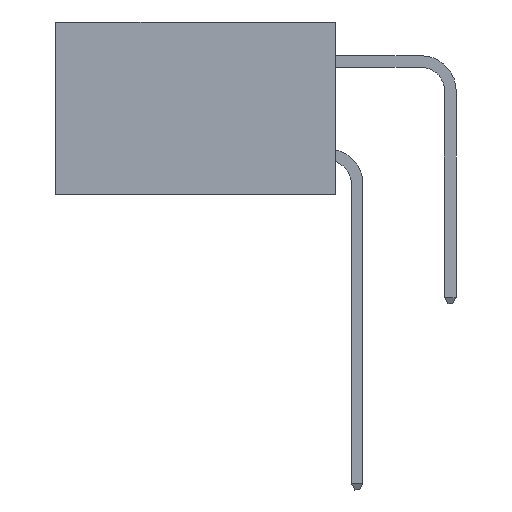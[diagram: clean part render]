
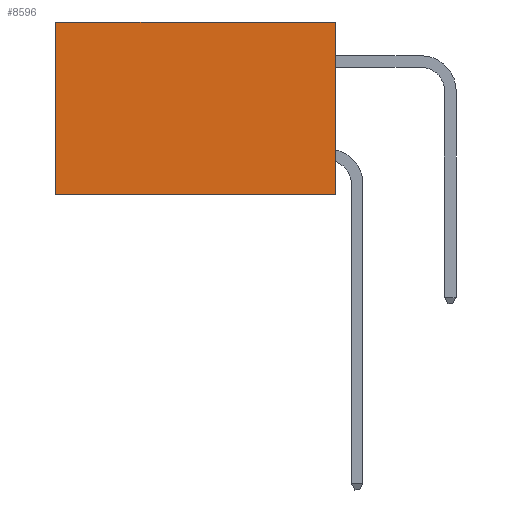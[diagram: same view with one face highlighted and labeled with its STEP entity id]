
A CAD part, left-side view. The second image highlights one B-rep face of the part: STEP entity #8596.
In plain terms, the highlighted planar face has unit normal (-1, 0, 0).
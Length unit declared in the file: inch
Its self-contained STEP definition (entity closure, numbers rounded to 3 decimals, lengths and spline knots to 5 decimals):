
#71 = DIRECTION ( 'NONE',  ( 0., 0., -1. ) ) ;
#148 = CARTESIAN_POINT ( 'NONE',  ( 0.2875, 0.6, 0. ) ) ;
#762 = LINE ( 'NONE', #14787, #14325 ) ;
#1506 = VERTEX_POINT ( 'NONE', #148 ) ;
#1534 = VECTOR ( 'NONE', #71, 39.37008 ) ;
#1707 = VERTEX_POINT ( 'NONE', #6057 ) ;
#3510 = EDGE_CURVE ( 'NONE', #1707, #11016, #5150, .T. ) ;
#3944 = FACE_OUTER_BOUND ( 'NONE', #10001, .T. ) ;
#4393 = ORIENTED_EDGE ( 'NONE', *, *, #6780, .T. ) ;
#4537 = DIRECTION ( 'NONE',  ( 0., 1., 0. ) ) ;
#4544 = VERTEX_POINT ( 'NONE', #5173 ) ;
#4645 = CARTESIAN_POINT ( 'NONE',  ( 0.2875, 0., 0. ) ) ;
#5020 = DIRECTION ( 'NONE',  ( 0., 0., -1. ) ) ;
#5150 = LINE ( 'NONE', #6116, #1534 ) ;
#5173 = CARTESIAN_POINT ( 'NONE',  ( 0.2875, 0.6, -0.37 ) ) ;
#6057 = CARTESIAN_POINT ( 'NONE',  ( 0.2875, 0., 0. ) ) ;
#6116 = CARTESIAN_POINT ( 'NONE',  ( 0.2875, 0., 0. ) ) ;
#6780 = EDGE_CURVE ( 'NONE', #1506, #4544, #16560, .T. ) ;
#7019 = LINE ( 'NONE', #7285, #16296 ) ;
#7285 = CARTESIAN_POINT ( 'NONE',  ( 0.2875, 0., -0.37 ) ) ;
#7332 = DIRECTION ( 'NONE',  ( 0., 0., -1. ) ) ;
#7420 = ORIENTED_EDGE ( 'NONE', *, *, #14141, .F. ) ;
#7575 = ORIENTED_EDGE ( 'NONE', *, *, #16465, .T. ) ;
#8430 = CARTESIAN_POINT ( 'NONE',  ( 0.2875, 0., -0.37 ) ) ;
#8596 = ADVANCED_FACE ( 'NONE', ( #3944 ), #13722, .F. ) ;
#9917 = DIRECTION ( 'NONE',  ( 0., 1., 0. ) ) ;
#9988 = AXIS2_PLACEMENT_3D ( 'NONE', #4645, #14939, #7332 ) ;
#10001 = EDGE_LOOP ( 'NONE', ( #4393, #7420, #12402, #7575 ) ) ;
#11016 = VERTEX_POINT ( 'NONE', #8430 ) ;
#12402 = ORIENTED_EDGE ( 'NONE', *, *, #3510, .F. ) ;
#13722 = PLANE ( 'NONE',  #9988 ) ;
#13724 = CARTESIAN_POINT ( 'NONE',  ( 0.2875, 0.6, 0. ) ) ;
#13758 = VECTOR ( 'NONE', #5020, 39.37008 ) ;
#14141 = EDGE_CURVE ( 'NONE', #11016, #4544, #7019, .T. ) ;
#14325 = VECTOR ( 'NONE', #4537, 39.37008 ) ;
#14787 = CARTESIAN_POINT ( 'NONE',  ( 0.2875, 0., 0. ) ) ;
#14939 = DIRECTION ( 'NONE',  ( 1., 0., 0. ) ) ;
#16296 = VECTOR ( 'NONE', #9917, 39.37008 ) ;
#16465 = EDGE_CURVE ( 'NONE', #1707, #1506, #762, .T. ) ;
#16560 = LINE ( 'NONE', #13724, #13758 ) ;
